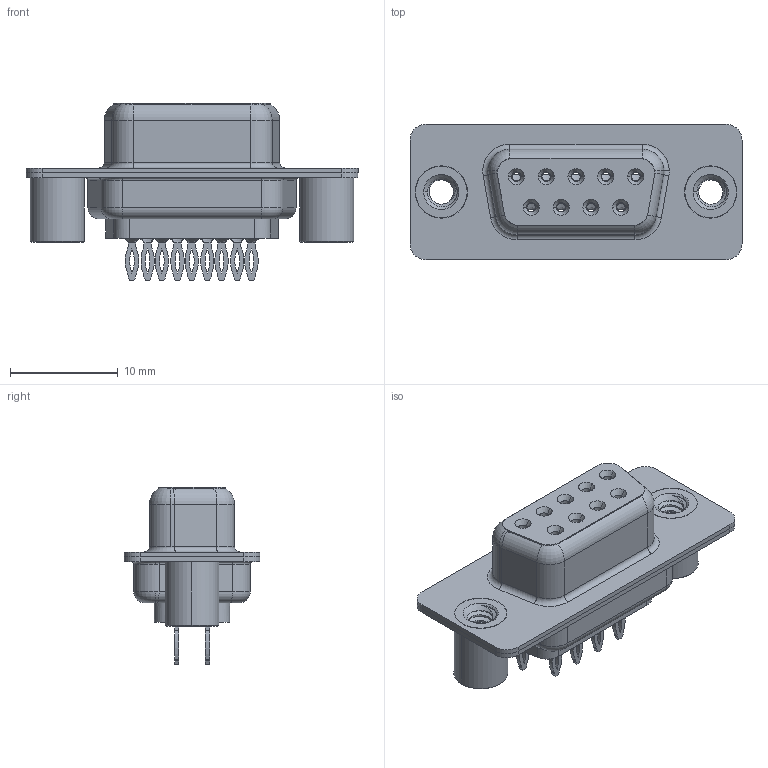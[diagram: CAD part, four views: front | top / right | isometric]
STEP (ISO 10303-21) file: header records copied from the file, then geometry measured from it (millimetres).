
FILE_DESCRIPTION (( 'STEP AP203' ), '1' );
FILE_NAME ('628-009-226-049.STEP', '2020-07-13T19:00:55', ( '' ), ( '' ), 'SwSTEP 2.0', 'SolidWorks 2020', '' );
FILE_SCHEMA (( 'CONFIG_CONTROL_DESIGN' ));
Length unit declared in the file: millimetre
Products named in the file (7): 628 Housing_09 LP; 628 Shell Front_09 Contacts; 628-009-226-049; 628 Shell Rear_09 Contacts; 628 4-40 Threaded Standoff BS; 628 Contact Row 2_26L; 628 Contact Row 1_26L
Assembly tree (14 placements, depth 2):
  628-009-226-049
    628 Housing_09 LP
    628 Shell Front_09 Contacts
    628 Shell Rear_09 Contacts
    628 Contact Row 1_26L  x5
    628 Contact Row 2_26L  x4
    628 4-40 Threaded Standoff BS  x2
Bounding box: 30.8 x 12.6 x 16.45 mm (x, y, z)
Volume: 1854 mm3; surface area: 4667.7 mm2
Topology: 14 solids, 14 shells, 1210 faces, 3035 edges, 1891 vertices
Faces by surface type: cylinder 400, plane 310, bspline 222, torus 219, cone 59
Entity records: 20475 total; most frequent: CARTESIAN_POINT 6746, DIRECTION 2711, ORIENTED_EDGE 2680, EDGE_CURVE 1340, AXIS2_PLACEMENT_3D 1106, VERTEX_POINT 838, EDGE_LOOP 622, CIRCLE 590
